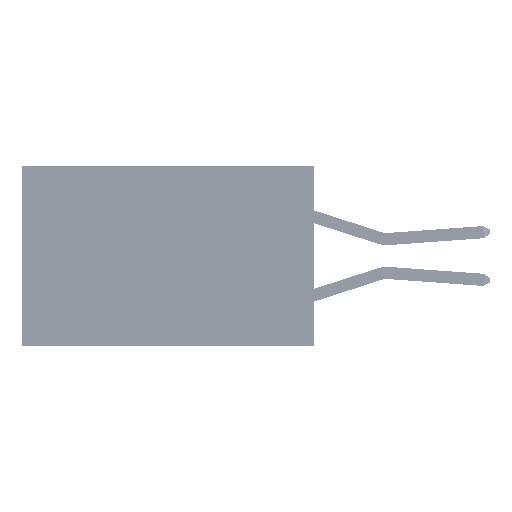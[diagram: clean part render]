
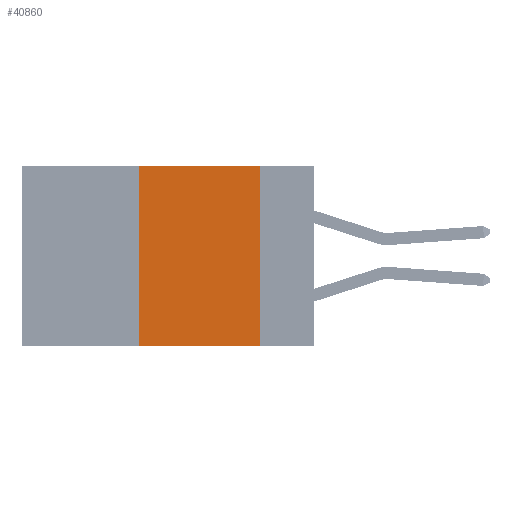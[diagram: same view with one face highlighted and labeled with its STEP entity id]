
A CAD part, left-side view. The second image highlights one B-rep face of the part: STEP entity #40860.
In plain terms, the highlighted planar face has unit normal (-1, 0, 0).
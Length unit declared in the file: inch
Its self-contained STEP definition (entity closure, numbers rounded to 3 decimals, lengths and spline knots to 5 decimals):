
#3381 = EDGE_CURVE ( 'NONE', #10656, #23292, #39590, .T. ) ;
#3834 = ORIENTED_EDGE ( 'NONE', *, *, #3381, .T. ) ;
#5577 = CARTESIAN_POINT ( 'NONE',  ( 0., 0.11, 0. ) ) ;
#6724 = CARTESIAN_POINT ( 'NONE',  ( 0., 0.36, 0. ) ) ;
#7708 = DIRECTION ( 'NONE',  ( 0., 0., -1. ) ) ;
#8065 = DIRECTION ( 'NONE',  ( 0., 0., -1. ) ) ;
#8388 = CARTESIAN_POINT ( 'NONE',  ( 0., 0.36, 0. ) ) ;
#8958 = VECTOR ( 'NONE', #44024, 39.37008 ) ;
#10656 = VERTEX_POINT ( 'NONE', #22080 ) ;
#11395 = DIRECTION ( 'NONE',  ( 1., 0., 0. ) ) ;
#12162 = FACE_OUTER_BOUND ( 'NONE', #18663, .T. ) ;
#12257 = AXIS2_PLACEMENT_3D ( 'NONE', #28121, #11395, #7708 ) ;
#12804 = CARTESIAN_POINT ( 'NONE',  ( 0., 0.6, 0. ) ) ;
#15582 = PLANE ( 'NONE',  #12257 ) ;
#16742 = LINE ( 'NONE', #12804, #8958 ) ;
#17858 = ORIENTED_EDGE ( 'NONE', *, *, #27229, .F. ) ;
#18663 = EDGE_LOOP ( 'NONE', ( #48076, #19794, #17858, #3834 ) ) ;
#19647 = VECTOR ( 'NONE', #8065, 39.37008 ) ;
#19794 = ORIENTED_EDGE ( 'NONE', *, *, #41281, .F. ) ;
#22080 = CARTESIAN_POINT ( 'NONE',  ( 0., 0.36, -0.37 ) ) ;
#23272 = VERTEX_POINT ( 'NONE', #6724 ) ;
#23292 = VERTEX_POINT ( 'NONE', #50518 ) ;
#24612 = LINE ( 'NONE', #8388, #32967 ) ;
#27229 = EDGE_CURVE ( 'NONE', #10656, #23272, #24612, .T. ) ;
#27591 = EDGE_CURVE ( 'NONE', #51528, #23292, #31649, .T. ) ;
#28121 = CARTESIAN_POINT ( 'NONE',  ( 0., 0.6, 0. ) ) ;
#28284 = CARTESIAN_POINT ( 'NONE',  ( 0., 0.6, -0.37 ) ) ;
#31649 = LINE ( 'NONE', #47683, #19647 ) ;
#32967 = VECTOR ( 'NONE', #43807, 39.37008 ) ;
#36046 = VECTOR ( 'NONE', #43801, 39.37008 ) ;
#39590 = LINE ( 'NONE', #28284, #36046 ) ;
#40860 = ADVANCED_FACE ( 'NONE', ( #12162 ), #15582, .F. ) ;
#41281 = EDGE_CURVE ( 'NONE', #23272, #51528, #16742, .T. ) ;
#43801 = DIRECTION ( 'NONE',  ( 0., -1., 0. ) ) ;
#43807 = DIRECTION ( 'NONE',  ( 0., 0., 1. ) ) ;
#44024 = DIRECTION ( 'NONE',  ( 0., -1., 0. ) ) ;
#47683 = CARTESIAN_POINT ( 'NONE',  ( 0., 0.11, 0. ) ) ;
#48076 = ORIENTED_EDGE ( 'NONE', *, *, #27591, .F. ) ;
#50518 = CARTESIAN_POINT ( 'NONE',  ( 0., 0.11, -0.37 ) ) ;
#51528 = VERTEX_POINT ( 'NONE', #5577 ) ;
